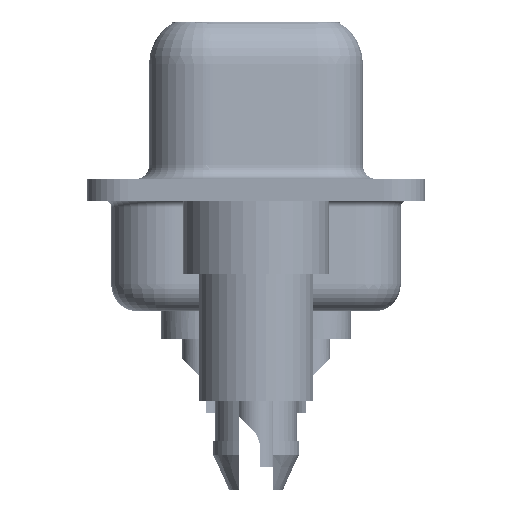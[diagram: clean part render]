
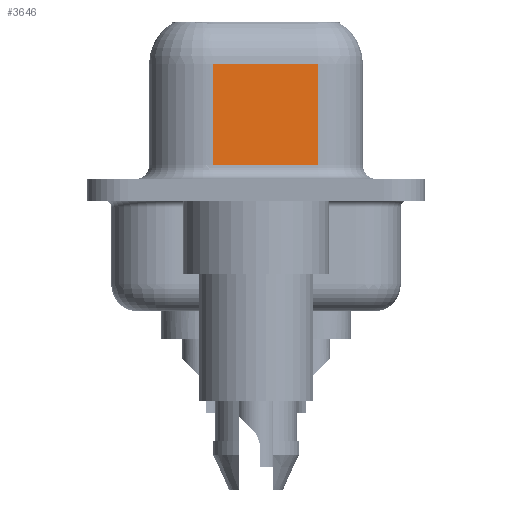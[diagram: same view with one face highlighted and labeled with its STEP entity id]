
A CAD part, left-side view. The second image highlights one B-rep face of the part: STEP entity #3646.
In plain terms, the highlighted planar face has unit normal (-0.985, -0.174, 0).
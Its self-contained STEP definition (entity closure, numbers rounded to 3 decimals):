
#1122 = CARTESIAN_POINT ( 'NONE',  ( 5.068, -2.297, 4.65 ) ) ;
#1993 = LINE ( 'NONE', #14186, #22865 ) ;
#3646 = ADVANCED_FACE ( 'NONE', ( #34367 ), #19830, .F. ) ;
#3657 = VECTOR ( 'NONE', #22464, 1000. ) ;
#3912 = CARTESIAN_POINT ( 'NONE',  ( 5.068, -2.297, 4.65 ) ) ;
#4459 = VERTEX_POINT ( 'NONE', #25450 ) ;
#5105 = CARTESIAN_POINT ( 'NONE',  ( 4.38, 1.603, 6.4 ) ) ;
#5641 = CARTESIAN_POINT ( 'NONE',  ( 5.068, -2.297, 0.9 ) ) ;
#5834 = EDGE_CURVE ( 'NONE', #11205, #4459, #9819, .T. ) ;
#8321 = ORIENTED_EDGE ( 'NONE', *, *, #13656, .F. ) ;
#8501 = VECTOR ( 'NONE', #17846, 1000. ) ;
#9819 = LINE ( 'NONE', #3912, #13016 ) ;
#10938 = DIRECTION ( 'NONE',  ( 0.985, 0.174, 0. ) ) ;
#11205 = VERTEX_POINT ( 'NONE', #1122 ) ;
#13016 = VECTOR ( 'NONE', #27358, 1000. ) ;
#13656 = EDGE_CURVE ( 'NONE', #11205, #23151, #1993, .T. ) ;
#14186 = CARTESIAN_POINT ( 'NONE',  ( 5.068, -2.297, 6.4 ) ) ;
#15220 = ORIENTED_EDGE ( 'NONE', *, *, #5834, .T. ) ;
#17207 = ORIENTED_EDGE ( 'NONE', *, *, #36641, .T. ) ;
#17601 = CARTESIAN_POINT ( 'NONE',  ( 5.068, -2.297, 0.9 ) ) ;
#17846 = DIRECTION ( 'NONE',  ( 0.174, -0.985, 0. ) ) ;
#18648 = ORIENTED_EDGE ( 'NONE', *, *, #30296, .T. ) ;
#19830 = PLANE ( 'NONE',  #20867 ) ;
#20867 = AXIS2_PLACEMENT_3D ( 'NONE', #23741, #10938, #23543 ) ;
#22464 = DIRECTION ( 'NONE',  ( 0., 0., -1. ) ) ;
#22865 = VECTOR ( 'NONE', #25847, 1000. ) ;
#23018 = EDGE_LOOP ( 'NONE', ( #8321, #15220, #17207, #18648 ) ) ;
#23151 = VERTEX_POINT ( 'NONE', #17601 ) ;
#23543 = DIRECTION ( 'NONE',  ( -0.174, 0.985, 0. ) ) ;
#23741 = CARTESIAN_POINT ( 'NONE',  ( 5.068, -2.297, 6.4 ) ) ;
#25450 = CARTESIAN_POINT ( 'NONE',  ( 4.38, 1.603, 4.65 ) ) ;
#25847 = DIRECTION ( 'NONE',  ( 0., 0., -1. ) ) ;
#27358 = DIRECTION ( 'NONE',  ( -0.174, 0.985, 0. ) ) ;
#30021 = VERTEX_POINT ( 'NONE', #30294 ) ;
#30294 = CARTESIAN_POINT ( 'NONE',  ( 4.38, 1.603, 0.9 ) ) ;
#30296 = EDGE_CURVE ( 'NONE', #30021, #23151, #38481, .T. ) ;
#32083 = LINE ( 'NONE', #5105, #3657 ) ;
#34367 = FACE_OUTER_BOUND ( 'NONE', #23018, .T. ) ;
#36641 = EDGE_CURVE ( 'NONE', #4459, #30021, #32083, .T. ) ;
#38481 = LINE ( 'NONE', #5641, #8501 ) ;
